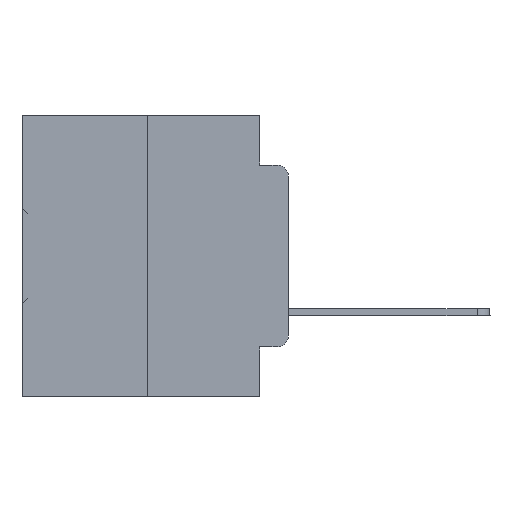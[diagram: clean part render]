
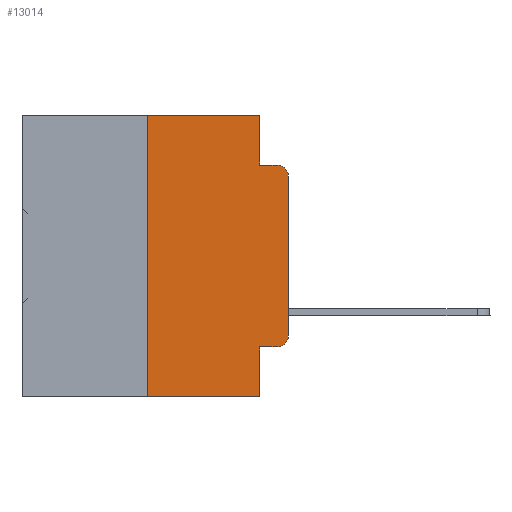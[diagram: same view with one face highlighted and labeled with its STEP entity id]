
A CAD part, left-side view. The second image highlights one B-rep face of the part: STEP entity #13014.
In plain terms, the highlighted planar face has unit normal (-1, 0, 0).
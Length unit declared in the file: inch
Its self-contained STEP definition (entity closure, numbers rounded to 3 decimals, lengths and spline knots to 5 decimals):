
#174 = ORIENTED_EDGE ( 'NONE', *, *, #21428, .F. ) ;
#263 = VECTOR ( 'NONE', #5549, 39.37008 ) ;
#268 = CARTESIAN_POINT ( 'NONE',  ( 0., 0.051, 0. ) ) ;
#322 = CARTESIAN_POINT ( 'NONE',  ( 0., 0.051, 0. ) ) ;
#1477 = ORIENTED_EDGE ( 'NONE', *, *, #25443, .F. ) ;
#1633 = VERTEX_POINT ( 'NONE', #11661 ) ;
#2547 = EDGE_CURVE ( 'NONE', #21444, #26035, #16031, .T. ) ;
#2741 = CARTESIAN_POINT ( 'NONE',  ( 0., 0.051, -0.4115 ) ) ;
#3738 = LINE ( 'NONE', #22890, #25412 ) ;
#3761 = ORIENTED_EDGE ( 'NONE', *, *, #11749, .F. ) ;
#4009 = CARTESIAN_POINT ( 'NONE',  ( 0., 0.25, -0.5 ) ) ;
#4237 = VECTOR ( 'NONE', #27356, 39.37008 ) ;
#4771 = ORIENTED_EDGE ( 'NONE', *, *, #35307, .T. ) ;
#5012 = EDGE_CURVE ( 'NONE', #10767, #10714, #13623, .T. ) ;
#5207 = ORIENTED_EDGE ( 'NONE', *, *, #12722, .F. ) ;
#5549 = DIRECTION ( 'NONE',  ( 0., 0., -1. ) ) ;
#5795 = PLANE ( 'NONE',  #36141 ) ;
#6005 = DIRECTION ( 'NONE',  ( 0., 0., -1. ) ) ;
#6245 = DIRECTION ( 'NONE',  ( 0., 0., 1. ) ) ;
#6338 = VECTOR ( 'NONE', #17674, 39.37008 ) ;
#6636 = VECTOR ( 'NONE', #18806, 39.37008 ) ;
#7209 = CARTESIAN_POINT ( 'NONE',  ( 0., 0.473, -0.5 ) ) ;
#8191 = VECTOR ( 'NONE', #6245, 39.37008 ) ;
#8632 = DIRECTION ( 'NONE',  ( 1., 0., 0. ) ) ;
#8876 = DIRECTION ( 'NONE',  ( 0., -1., 0. ) ) ;
#9648 = CIRCLE ( 'NONE', #15837, 0.02 ) ;
#10318 = EDGE_CURVE ( 'NONE', #20050, #10767, #22824, .T. ) ;
#10714 = VERTEX_POINT ( 'NONE', #34901 ) ;
#10767 = VERTEX_POINT ( 'NONE', #34652 ) ;
#11335 = EDGE_CURVE ( 'NONE', #20050, #26035, #21445, .T. ) ;
#11487 = DIRECTION ( 'NONE',  ( 0., 0., -1. ) ) ;
#11661 = CARTESIAN_POINT ( 'NONE',  ( 0., 0., -0.1085 ) ) ;
#11749 = EDGE_CURVE ( 'NONE', #20051, #22291, #31560, .T. ) ;
#12238 = DIRECTION ( 'NONE',  ( 0., 0., -1. ) ) ;
#12440 = ORIENTED_EDGE ( 'NONE', *, *, #10318, .T. ) ;
#12722 = EDGE_CURVE ( 'NONE', #21444, #17641, #15743, .T. ) ;
#13014 = ADVANCED_FACE ( 'NONE', ( #18332 ), #5795, .F. ) ;
#13623 = CIRCLE ( 'NONE', #20645, 0.02 ) ;
#15572 = ORIENTED_EDGE ( 'NONE', *, *, #30286, .T. ) ;
#15743 = LINE ( 'NONE', #17248, #8191 ) ;
#15792 = DIRECTION ( 'NONE',  ( 0., -1., 0. ) ) ;
#15837 = AXIS2_PLACEMENT_3D ( 'NONE', #23225, #29161, #12238 ) ;
#16031 = LINE ( 'NONE', #7209, #32848 ) ;
#17248 = CARTESIAN_POINT ( 'NONE',  ( 0., 0.25, 0. ) ) ;
#17280 = CARTESIAN_POINT ( 'NONE',  ( 0., 0.02, -0.3915 ) ) ;
#17641 = VERTEX_POINT ( 'NONE', #33420 ) ;
#17674 = DIRECTION ( 'NONE',  ( 0., 0., -1. ) ) ;
#18332 = FACE_OUTER_BOUND ( 'NONE', #31496, .T. ) ;
#18806 = DIRECTION ( 'NONE',  ( 0., 0., 1. ) ) ;
#20050 = VERTEX_POINT ( 'NONE', #2741 ) ;
#20051 = VERTEX_POINT ( 'NONE', #31082 ) ;
#20645 = AXIS2_PLACEMENT_3D ( 'NONE', #17280, #28874, #6005 ) ;
#21428 = EDGE_CURVE ( 'NONE', #17641, #24050, #3738, .T. ) ;
#21444 = VERTEX_POINT ( 'NONE', #4009 ) ;
#21445 = LINE ( 'NONE', #322, #6338 ) ;
#22291 = VERTEX_POINT ( 'NONE', #35805 ) ;
#22824 = LINE ( 'NONE', #24274, #4237 ) ;
#22890 = CARTESIAN_POINT ( 'NONE',  ( 0., 0.473, 0. ) ) ;
#23225 = CARTESIAN_POINT ( 'NONE',  ( 0., 0.02, -0.1085 ) ) ;
#23815 = DIRECTION ( 'NONE',  ( 0., -1., 0. ) ) ;
#24050 = VERTEX_POINT ( 'NONE', #268 ) ;
#24274 = CARTESIAN_POINT ( 'NONE',  ( 0., 0.051, -0.4115 ) ) ;
#25315 = CARTESIAN_POINT ( 'NONE',  ( 0., 0.051, 0. ) ) ;
#25412 = VECTOR ( 'NONE', #8876, 39.37008 ) ;
#25443 = EDGE_CURVE ( 'NONE', #24050, #20051, #30441, .T. ) ;
#25551 = CARTESIAN_POINT ( 'NONE',  ( 0., 0.473, 0. ) ) ;
#25580 = CARTESIAN_POINT ( 'NONE',  ( 0., 0.051, -0.5 ) ) ;
#26035 = VERTEX_POINT ( 'NONE', #25580 ) ;
#26102 = LINE ( 'NONE', #30423, #6636 ) ;
#27356 = DIRECTION ( 'NONE',  ( 0., -1., 0. ) ) ;
#28874 = DIRECTION ( 'NONE',  ( -1., 0., 0. ) ) ;
#29161 = DIRECTION ( 'NONE',  ( -1., 0., 0. ) ) ;
#30286 = EDGE_CURVE ( 'NONE', #1633, #22291, #9648, .T. ) ;
#30335 = ORIENTED_EDGE ( 'NONE', *, *, #2547, .T. ) ;
#30423 = CARTESIAN_POINT ( 'NONE',  ( 0., 0., 0. ) ) ;
#30441 = LINE ( 'NONE', #25315, #263 ) ;
#31082 = CARTESIAN_POINT ( 'NONE',  ( 0., 0.051, -0.0885 ) ) ;
#31496 = EDGE_LOOP ( 'NONE', ( #4771, #15572, #3761, #1477, #174, #5207, #30335, #33336, #12440, #34503 ) ) ;
#31560 = LINE ( 'NONE', #31613, #35582 ) ;
#31613 = CARTESIAN_POINT ( 'NONE',  ( 0., 0.051, -0.0885 ) ) ;
#32848 = VECTOR ( 'NONE', #15792, 39.37008 ) ;
#33336 = ORIENTED_EDGE ( 'NONE', *, *, #11335, .F. ) ;
#33420 = CARTESIAN_POINT ( 'NONE',  ( 0., 0.25, 0. ) ) ;
#34503 = ORIENTED_EDGE ( 'NONE', *, *, #5012, .T. ) ;
#34652 = CARTESIAN_POINT ( 'NONE',  ( 0., 0.02, -0.4115 ) ) ;
#34901 = CARTESIAN_POINT ( 'NONE',  ( 0., 0., -0.3915 ) ) ;
#35307 = EDGE_CURVE ( 'NONE', #10714, #1633, #26102, .T. ) ;
#35582 = VECTOR ( 'NONE', #23815, 39.37008 ) ;
#35805 = CARTESIAN_POINT ( 'NONE',  ( 0., 0.02, -0.0885 ) ) ;
#36141 = AXIS2_PLACEMENT_3D ( 'NONE', #25551, #8632, #11487 ) ;
